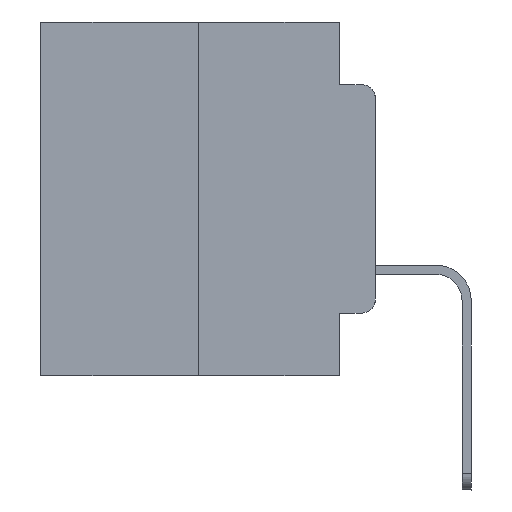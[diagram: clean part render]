
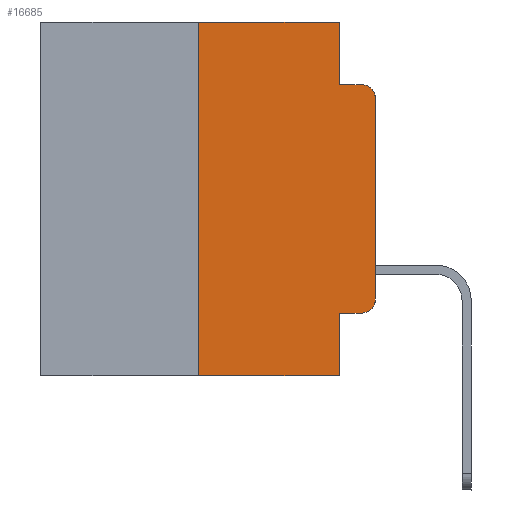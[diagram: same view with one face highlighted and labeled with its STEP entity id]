
A CAD part, left-side view. The second image highlights one B-rep face of the part: STEP entity #16685.
In plain terms, the highlighted planar face has unit normal (-1, 0, 0).
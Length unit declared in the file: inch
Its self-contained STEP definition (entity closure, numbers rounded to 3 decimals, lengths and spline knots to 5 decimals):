
#222 = EDGE_CURVE ( 'NONE', #21020, #2491, #14080, .T. ) ;
#236 = ORIENTED_EDGE ( 'NONE', *, *, #21330, .F. ) ;
#1192 = AXIS2_PLACEMENT_3D ( 'NONE', #1560, #5733, #9671 ) ;
#1560 = CARTESIAN_POINT ( 'NONE',  ( 0., 0.02, -0.1085 ) ) ;
#1628 = DIRECTION ( 'NONE',  ( 0., -1., 0. ) ) ;
#2112 = EDGE_CURVE ( 'NONE', #13152, #21020, #14356, .T. ) ;
#2491 = VERTEX_POINT ( 'NONE', #19561 ) ;
#2633 = DIRECTION ( 'NONE',  ( 0., 0., -1. ) ) ;
#3006 = VECTOR ( 'NONE', #22078, 39.37008 ) ;
#3258 = DIRECTION ( 'NONE',  ( 0., -1., 0. ) ) ;
#3504 = VERTEX_POINT ( 'NONE', #16307 ) ;
#4653 = CARTESIAN_POINT ( 'NONE',  ( 0., 0.051, -0.0885 ) ) ;
#4890 = CARTESIAN_POINT ( 'NONE',  ( 0., 0.25, 0. ) ) ;
#5215 = LINE ( 'NONE', #15970, #3006 ) ;
#5373 = CARTESIAN_POINT ( 'NONE',  ( 0., 0.473, -0.5 ) ) ;
#5733 = DIRECTION ( 'NONE',  ( -1., 0., 0. ) ) ;
#6257 = EDGE_CURVE ( 'NONE', #20412, #11795, #5215, .T. ) ;
#6450 = EDGE_CURVE ( 'NONE', #21950, #2491, #24535, .T. ) ;
#6746 = ORIENTED_EDGE ( 'NONE', *, *, #20071, .T. ) ;
#7306 = VECTOR ( 'NONE', #3258, 39.37008 ) ;
#7360 = ORIENTED_EDGE ( 'NONE', *, *, #2112, .T. ) ;
#7624 = LINE ( 'NONE', #5373, #7306 ) ;
#7762 = EDGE_LOOP ( 'NONE', ( #7360, #8287, #11333, #14803, #13836, #8873, #13233, #236, #12978, #6746 ) ) ;
#8060 = DIRECTION ( 'NONE',  ( -1., 0., 0. ) ) ;
#8287 = ORIENTED_EDGE ( 'NONE', *, *, #222, .T. ) ;
#8783 = VERTEX_POINT ( 'NONE', #15378 ) ;
#8873 = ORIENTED_EDGE ( 'NONE', *, *, #8961, .F. ) ;
#8961 = EDGE_CURVE ( 'NONE', #18204, #20412, #25945, .T. ) ;
#8971 = VECTOR ( 'NONE', #24922, 39.37008 ) ;
#9671 = DIRECTION ( 'NONE',  ( 0., 0., -1. ) ) ;
#10207 = VECTOR ( 'NONE', #16221, 39.37008 ) ;
#10667 = CARTESIAN_POINT ( 'NONE',  ( 0., 0.051, -0.4115 ) ) ;
#10757 = CARTESIAN_POINT ( 'NONE',  ( 0., 0.051, 0. ) ) ;
#10819 = CARTESIAN_POINT ( 'NONE',  ( 0., 0.25, 0. ) ) ;
#11333 = ORIENTED_EDGE ( 'NONE', *, *, #6450, .F. ) ;
#11408 = CARTESIAN_POINT ( 'NONE',  ( 0., 0.25, -0.5 ) ) ;
#11461 = AXIS2_PLACEMENT_3D ( 'NONE', #18356, #8060, #22248 ) ;
#11688 = CIRCLE ( 'NONE', #11461, 0.02 ) ;
#11709 = PLANE ( 'NONE',  #20592 ) ;
#11795 = VERTEX_POINT ( 'NONE', #23281 ) ;
#12491 = EDGE_CURVE ( 'NONE', #18204, #8783, #7624, .T. ) ;
#12871 = LINE ( 'NONE', #23854, #17622 ) ;
#12978 = ORIENTED_EDGE ( 'NONE', *, *, #26051, .T. ) ;
#13152 = VERTEX_POINT ( 'NONE', #16123 ) ;
#13233 = ORIENTED_EDGE ( 'NONE', *, *, #12491, .T. ) ;
#13245 = LINE ( 'NONE', #13771, #25610 ) ;
#13590 = DIRECTION ( 'NONE',  ( 0., 0., -1. ) ) ;
#13738 = DIRECTION ( 'NONE',  ( 0., 0., -1. ) ) ;
#13771 = CARTESIAN_POINT ( 'NONE',  ( 0., 0.051, 0. ) ) ;
#13836 = ORIENTED_EDGE ( 'NONE', *, *, #6257, .F. ) ;
#14080 = CIRCLE ( 'NONE', #1192, 0.02 ) ;
#14217 = EDGE_CURVE ( 'NONE', #11795, #21950, #13245, .T. ) ;
#14356 = LINE ( 'NONE', #16507, #10207 ) ;
#14803 = ORIENTED_EDGE ( 'NONE', *, *, #14217, .F. ) ;
#14901 = DIRECTION ( 'NONE',  ( 0., 0., 1. ) ) ;
#15150 = CARTESIAN_POINT ( 'NONE',  ( 0., 0.051, -0.0885 ) ) ;
#15378 = CARTESIAN_POINT ( 'NONE',  ( 0., 0.051, -0.5 ) ) ;
#15689 = DIRECTION ( 'NONE',  ( 1., 0., 0. ) ) ;
#15970 = CARTESIAN_POINT ( 'NONE',  ( 0., 0.473, 0. ) ) ;
#16095 = VECTOR ( 'NONE', #2633, 39.37008 ) ;
#16123 = CARTESIAN_POINT ( 'NONE',  ( 0., 0., -0.3915 ) ) ;
#16221 = DIRECTION ( 'NONE',  ( 0., 0., 1. ) ) ;
#16307 = CARTESIAN_POINT ( 'NONE',  ( 0., 0.02, -0.4115 ) ) ;
#16507 = CARTESIAN_POINT ( 'NONE',  ( 0., 0., 0. ) ) ;
#16685 = ADVANCED_FACE ( 'NONE', ( #19464 ), #11709, .F. ) ;
#17375 = LINE ( 'NONE', #10757, #16095 ) ;
#17622 = VECTOR ( 'NONE', #1628, 39.37008 ) ;
#18000 = CARTESIAN_POINT ( 'NONE',  ( 0., 0.473, 0. ) ) ;
#18204 = VERTEX_POINT ( 'NONE', #11408 ) ;
#18356 = CARTESIAN_POINT ( 'NONE',  ( 0., 0.02, -0.3915 ) ) ;
#19464 = FACE_OUTER_BOUND ( 'NONE', #7762, .T. ) ;
#19561 = CARTESIAN_POINT ( 'NONE',  ( 0., 0.02, -0.0885 ) ) ;
#20071 = EDGE_CURVE ( 'NONE', #3504, #13152, #11688, .T. ) ;
#20412 = VERTEX_POINT ( 'NONE', #4890 ) ;
#20592 = AXIS2_PLACEMENT_3D ( 'NONE', #18000, #15689, #13738 ) ;
#21020 = VERTEX_POINT ( 'NONE', #23718 ) ;
#21330 = EDGE_CURVE ( 'NONE', #25735, #8783, #17375, .T. ) ;
#21812 = VECTOR ( 'NONE', #14901, 39.37008 ) ;
#21950 = VERTEX_POINT ( 'NONE', #15150 ) ;
#22078 = DIRECTION ( 'NONE',  ( 0., -1., 0. ) ) ;
#22248 = DIRECTION ( 'NONE',  ( 0., 0., -1. ) ) ;
#23281 = CARTESIAN_POINT ( 'NONE',  ( 0., 0.051, 0. ) ) ;
#23718 = CARTESIAN_POINT ( 'NONE',  ( 0., 0., -0.1085 ) ) ;
#23854 = CARTESIAN_POINT ( 'NONE',  ( 0., 0.051, -0.4115 ) ) ;
#24535 = LINE ( 'NONE', #4653, #8971 ) ;
#24922 = DIRECTION ( 'NONE',  ( 0., -1., 0. ) ) ;
#25610 = VECTOR ( 'NONE', #13590, 39.37008 ) ;
#25735 = VERTEX_POINT ( 'NONE', #10667 ) ;
#25945 = LINE ( 'NONE', #10819, #21812 ) ;
#26051 = EDGE_CURVE ( 'NONE', #25735, #3504, #12871, .T. ) ;
